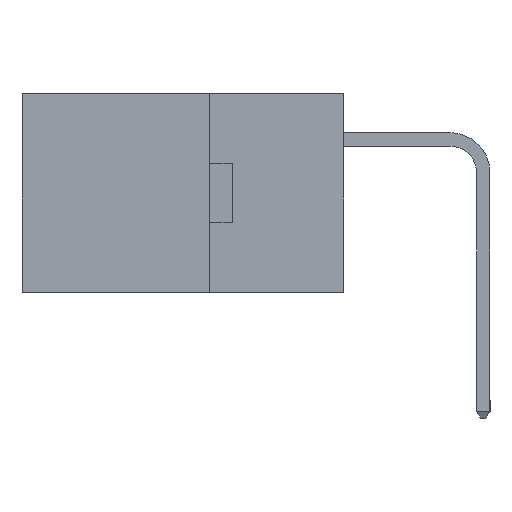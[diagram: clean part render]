
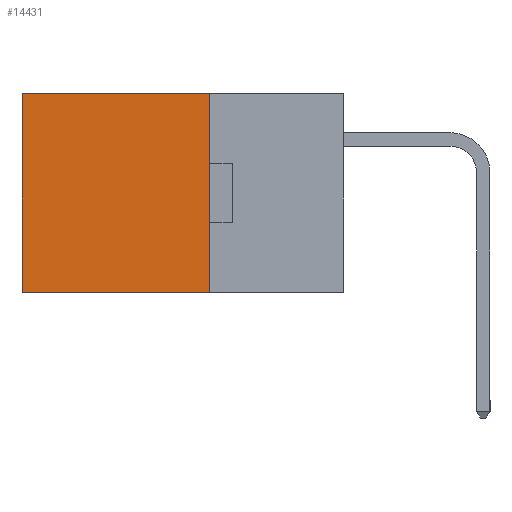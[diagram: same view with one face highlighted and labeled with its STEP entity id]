
A CAD part, left-side view. The second image highlights one B-rep face of the part: STEP entity #14431.
In plain terms, the highlighted planar face has unit normal (-1, 0, 0).
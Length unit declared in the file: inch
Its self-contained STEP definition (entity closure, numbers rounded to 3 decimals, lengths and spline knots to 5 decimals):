
#312 = CARTESIAN_POINT ( 'NONE',  ( 0.2615, 0.25, 0. ) ) ;
#1356 = EDGE_CURVE ( 'NONE', #17799, #17952, #26093, .T. ) ;
#2231 = CARTESIAN_POINT ( 'NONE',  ( 0.2615, 0.25, -0.37 ) ) ;
#2576 = DIRECTION ( 'NONE',  ( 0., 0., -1. ) ) ;
#2697 = CARTESIAN_POINT ( 'NONE',  ( 0.2615, 0.6, -0.37 ) ) ;
#3573 = CARTESIAN_POINT ( 'NONE',  ( 0.2615, 0.25, -0.37 ) ) ;
#3858 = CARTESIAN_POINT ( 'NONE',  ( 0.2615, 0.25, -0.37 ) ) ;
#3910 = CARTESIAN_POINT ( 'NONE',  ( 0.2615, 0.6, 0. ) ) ;
#4951 = VECTOR ( 'NONE', #11741, 39.37008 ) ;
#8793 = EDGE_CURVE ( 'NONE', #21503, #17952, #15504, .T. ) ;
#9071 = EDGE_CURVE ( 'NONE', #15345, #17799, #13895, .T. ) ;
#9686 = CARTESIAN_POINT ( 'NONE',  ( 0.2615, 0.25, -0.37 ) ) ;
#10700 = VECTOR ( 'NONE', #18838, 39.37008 ) ;
#11741 = DIRECTION ( 'NONE',  ( 0., 0., -1. ) ) ;
#12269 = DIRECTION ( 'NONE',  ( 1., 0., 0. ) ) ;
#12445 = EDGE_CURVE ( 'NONE', #15345, #21503, #15938, .T. ) ;
#13705 = ORIENTED_EDGE ( 'NONE', *, *, #12445, .F. ) ;
#13895 = LINE ( 'NONE', #21755, #18669 ) ;
#14431 = ADVANCED_FACE ( 'NONE', ( #19027 ), #18324, .F. ) ;
#14460 = ORIENTED_EDGE ( 'NONE', *, *, #8793, .F. ) ;
#15345 = VERTEX_POINT ( 'NONE', #312 ) ;
#15504 = LINE ( 'NONE', #2231, #10700 ) ;
#15938 = LINE ( 'NONE', #9686, #4951 ) ;
#16521 = ORIENTED_EDGE ( 'NONE', *, *, #1356, .T. ) ;
#17799 = VERTEX_POINT ( 'NONE', #3910 ) ;
#17921 = EDGE_LOOP ( 'NONE', ( #16521, #14460, #13705, #19975 ) ) ;
#17952 = VERTEX_POINT ( 'NONE', #18730 ) ;
#18324 = PLANE ( 'NONE',  #21669 ) ;
#18669 = VECTOR ( 'NONE', #23857, 39.37008 ) ;
#18730 = CARTESIAN_POINT ( 'NONE',  ( 0.2615, 0.6, -0.37 ) ) ;
#18838 = DIRECTION ( 'NONE',  ( 0., 1., 0. ) ) ;
#19027 = FACE_OUTER_BOUND ( 'NONE', #17921, .T. ) ;
#19975 = ORIENTED_EDGE ( 'NONE', *, *, #9071, .T. ) ;
#21503 = VERTEX_POINT ( 'NONE', #3573 ) ;
#21669 = AXIS2_PLACEMENT_3D ( 'NONE', #3858, #12269, #26649 ) ;
#21755 = CARTESIAN_POINT ( 'NONE',  ( 0.2615, 0.25, 0. ) ) ;
#23857 = DIRECTION ( 'NONE',  ( 0., 1., 0. ) ) ;
#25459 = VECTOR ( 'NONE', #2576, 39.37008 ) ;
#26093 = LINE ( 'NONE', #2697, #25459 ) ;
#26649 = DIRECTION ( 'NONE',  ( 0., 0., -1. ) ) ;
